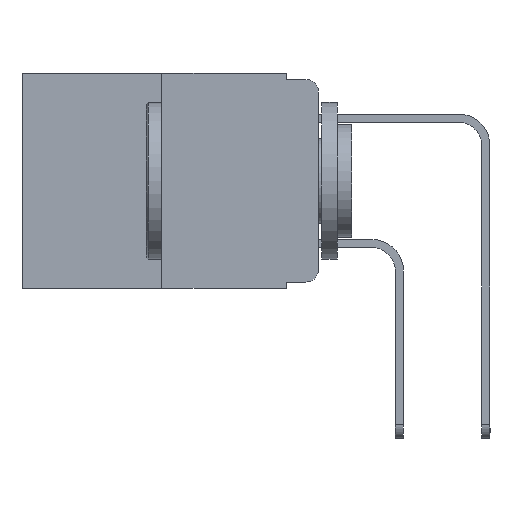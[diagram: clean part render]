
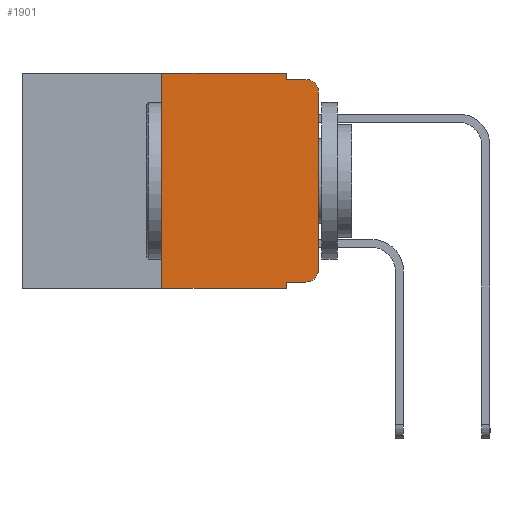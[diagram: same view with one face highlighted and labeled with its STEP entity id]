
A CAD part, left-side view. The second image highlights one B-rep face of the part: STEP entity #1901.
In plain terms, the highlighted planar face has unit normal (-1, 0, 0).
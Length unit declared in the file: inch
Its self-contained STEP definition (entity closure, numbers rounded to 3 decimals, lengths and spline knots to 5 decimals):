
#337 = VERTEX_POINT ( 'NONE', #11462 ) ;
#372 = CARTESIAN_POINT ( 'NONE',  ( 0., 0.02, -0.313 ) ) ;
#377 = VECTOR ( 'NONE', #17025, 39.37008 ) ;
#440 = CARTESIAN_POINT ( 'NONE',  ( 0., 0.473, -0.343 ) ) ;
#459 = VERTEX_POINT ( 'NONE', #1007 ) ;
#671 = LINE ( 'NONE', #2178, #377 ) ;
#1007 = CARTESIAN_POINT ( 'NONE',  ( 0., 0., -0.03 ) ) ;
#1712 = LINE ( 'NONE', #8843, #6180 ) ;
#1798 = CARTESIAN_POINT ( 'NONE',  ( 0., 0.02, -0.01 ) ) ;
#1865 = ORIENTED_EDGE ( 'NONE', *, *, #12195, .T. ) ;
#1901 = ADVANCED_FACE ( 'NONE', ( #2682 ), #13500, .F. ) ;
#2028 = VERTEX_POINT ( 'NONE', #1798 ) ;
#2074 = EDGE_CURVE ( 'NONE', #11441, #10640, #9820, .T. ) ;
#2178 = CARTESIAN_POINT ( 'NONE',  ( 0., 0.25, 0. ) ) ;
#2682 = FACE_OUTER_BOUND ( 'NONE', #9796, .T. ) ;
#3097 = VERTEX_POINT ( 'NONE', #4950 ) ;
#3136 = ORIENTED_EDGE ( 'NONE', *, *, #6243, .F. ) ;
#3361 = EDGE_CURVE ( 'NONE', #12773, #5902, #4464, .T. ) ;
#3395 = EDGE_CURVE ( 'NONE', #3097, #16160, #1712, .T. ) ;
#3474 = DIRECTION ( 'NONE',  ( 0., -1., 0. ) ) ;
#3587 = EDGE_CURVE ( 'NONE', #5902, #459, #5092, .T. ) ;
#4146 = ORIENTED_EDGE ( 'NONE', *, *, #5996, .T. ) ;
#4464 = CIRCLE ( 'NONE', #10174, 0.02 ) ;
#4470 = CARTESIAN_POINT ( 'NONE',  ( 0., 0.473, 0. ) ) ;
#4636 = CIRCLE ( 'NONE', #15495, 0.02 ) ;
#4950 = CARTESIAN_POINT ( 'NONE',  ( 0., 0.051, -0.333 ) ) ;
#5092 = LINE ( 'NONE', #11807, #6740 ) ;
#5227 = CARTESIAN_POINT ( 'NONE',  ( 0., 0.02, -0.03 ) ) ;
#5902 = VERTEX_POINT ( 'NONE', #15957 ) ;
#5996 = EDGE_CURVE ( 'NONE', #459, #2028, #4636, .T. ) ;
#6073 = VECTOR ( 'NONE', #15590, 39.37008 ) ;
#6084 = DIRECTION ( 'NONE',  ( 0., 0., -1. ) ) ;
#6180 = VECTOR ( 'NONE', #16722, 39.37008 ) ;
#6243 = EDGE_CURVE ( 'NONE', #337, #11441, #671, .T. ) ;
#6294 = EDGE_CURVE ( 'NONE', #10640, #15406, #15855, .T. ) ;
#6388 = VECTOR ( 'NONE', #9912, 39.37008 ) ;
#6740 = VECTOR ( 'NONE', #15827, 39.37008 ) ;
#7145 = CARTESIAN_POINT ( 'NONE',  ( 0., 0.051, -0.343 ) ) ;
#7345 = DIRECTION ( 'NONE',  ( -1., 0., 0. ) ) ;
#7346 = CARTESIAN_POINT ( 'NONE',  ( 0., 0.051, -0.333 ) ) ;
#8049 = DIRECTION ( 'NONE',  ( 0., 0., -1. ) ) ;
#8218 = ORIENTED_EDGE ( 'NONE', *, *, #12658, .T. ) ;
#8301 = CARTESIAN_POINT ( 'NONE',  ( 0., 0.473, 0. ) ) ;
#8424 = DIRECTION ( 'NONE',  ( 0., 0., -1. ) ) ;
#8534 = ORIENTED_EDGE ( 'NONE', *, *, #3395, .F. ) ;
#8657 = ORIENTED_EDGE ( 'NONE', *, *, #2074, .F. ) ;
#8843 = CARTESIAN_POINT ( 'NONE',  ( 0., 0.051, 0. ) ) ;
#9166 = ORIENTED_EDGE ( 'NONE', *, *, #13887, .F. ) ;
#9170 = VECTOR ( 'NONE', #13539, 39.37008 ) ;
#9414 = CARTESIAN_POINT ( 'NONE',  ( 0., 0.051, -0.01 ) ) ;
#9796 = EDGE_LOOP ( 'NONE', ( #16877, #4146, #9166, #16529, #8657, #3136, #8218, #8534, #1865, #10364 ) ) ;
#9820 = LINE ( 'NONE', #4470, #6388 ) ;
#9912 = DIRECTION ( 'NONE',  ( 0., -1., 0. ) ) ;
#10036 = VECTOR ( 'NONE', #12793, 39.37008 ) ;
#10126 = CARTESIAN_POINT ( 'NONE',  ( 0., 0.051, 0. ) ) ;
#10174 = AXIS2_PLACEMENT_3D ( 'NONE', #372, #7345, #6084 ) ;
#10364 = ORIENTED_EDGE ( 'NONE', *, *, #3361, .T. ) ;
#10491 = CARTESIAN_POINT ( 'NONE',  ( 0., 0.051, -0.01 ) ) ;
#10520 = CARTESIAN_POINT ( 'NONE',  ( 0., 0.02, -0.333 ) ) ;
#10605 = VECTOR ( 'NONE', #3474, 39.37008 ) ;
#10640 = VERTEX_POINT ( 'NONE', #14671 ) ;
#10666 = DIRECTION ( 'NONE',  ( -1., 0., 0. ) ) ;
#10681 = AXIS2_PLACEMENT_3D ( 'NONE', #8301, #14841, #8049 ) ;
#11441 = VERTEX_POINT ( 'NONE', #16037 ) ;
#11462 = CARTESIAN_POINT ( 'NONE',  ( 0., 0.25, -0.343 ) ) ;
#11807 = CARTESIAN_POINT ( 'NONE',  ( 0., 0., 0. ) ) ;
#12195 = EDGE_CURVE ( 'NONE', #3097, #12773, #12967, .T. ) ;
#12658 = EDGE_CURVE ( 'NONE', #337, #16160, #12680, .T. ) ;
#12680 = LINE ( 'NONE', #440, #10605 ) ;
#12773 = VERTEX_POINT ( 'NONE', #10520 ) ;
#12793 = DIRECTION ( 'NONE',  ( 0., -1., 0. ) ) ;
#12967 = LINE ( 'NONE', #7346, #10036 ) ;
#13500 = PLANE ( 'NONE',  #10681 ) ;
#13539 = DIRECTION ( 'NONE',  ( 0., -1., 0. ) ) ;
#13887 = EDGE_CURVE ( 'NONE', #15406, #2028, #16483, .T. ) ;
#14671 = CARTESIAN_POINT ( 'NONE',  ( 0., 0.051, 0. ) ) ;
#14841 = DIRECTION ( 'NONE',  ( 1., 0., 0. ) ) ;
#15406 = VERTEX_POINT ( 'NONE', #10491 ) ;
#15495 = AXIS2_PLACEMENT_3D ( 'NONE', #5227, #10666, #8424 ) ;
#15590 = DIRECTION ( 'NONE',  ( 0., 0., -1. ) ) ;
#15827 = DIRECTION ( 'NONE',  ( 0., 0., 1. ) ) ;
#15855 = LINE ( 'NONE', #10126, #6073 ) ;
#15957 = CARTESIAN_POINT ( 'NONE',  ( 0., 0., -0.313 ) ) ;
#16037 = CARTESIAN_POINT ( 'NONE',  ( 0., 0.25, 0. ) ) ;
#16160 = VERTEX_POINT ( 'NONE', #7145 ) ;
#16483 = LINE ( 'NONE', #9414, #9170 ) ;
#16529 = ORIENTED_EDGE ( 'NONE', *, *, #6294, .F. ) ;
#16722 = DIRECTION ( 'NONE',  ( 0., 0., -1. ) ) ;
#16877 = ORIENTED_EDGE ( 'NONE', *, *, #3587, .T. ) ;
#17025 = DIRECTION ( 'NONE',  ( 0., 0., 1. ) ) ;
